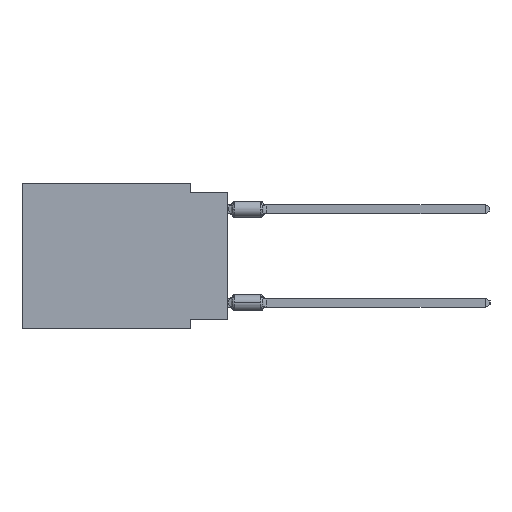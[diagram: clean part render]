
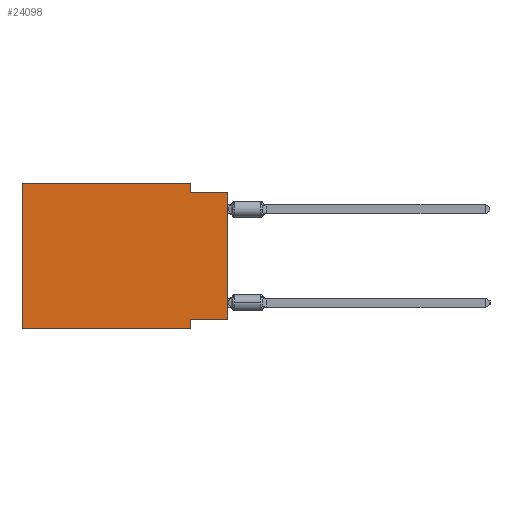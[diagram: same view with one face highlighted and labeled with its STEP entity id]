
A CAD part, left-side view. The second image highlights one B-rep face of the part: STEP entity #24098.
In plain terms, the highlighted planar face has unit normal (-1, 0, 0).
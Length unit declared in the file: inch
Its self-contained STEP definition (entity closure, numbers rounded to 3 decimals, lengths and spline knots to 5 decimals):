
#753 = DIRECTION ( 'NONE',  ( 0., 0., 1. ) ) ;
#770 = ORIENTED_EDGE ( 'NONE', *, *, #48475, .F. ) ;
#1580 = VERTEX_POINT ( 'NONE', #3614 ) ;
#2032 = DIRECTION ( 'NONE',  ( 0., 1., 0. ) ) ;
#2616 = CARTESIAN_POINT ( 'NONE',  ( 0., 0.1, 0. ) ) ;
#3614 = CARTESIAN_POINT ( 'NONE',  ( 0., 0.55, -0.39 ) ) ;
#4252 = ORIENTED_EDGE ( 'NONE', *, *, #18053, .T. ) ;
#5005 = CARTESIAN_POINT ( 'NONE',  ( 0., 0.55, 0. ) ) ;
#5665 = LINE ( 'NONE', #32160, #41641 ) ;
#5710 = ORIENTED_EDGE ( 'NONE', *, *, #48675, .F. ) ;
#7421 = CARTESIAN_POINT ( 'NONE',  ( 0., 0.1, 0. ) ) ;
#7492 = LINE ( 'NONE', #16198, #19968 ) ;
#7508 = VECTOR ( 'NONE', #34671, 39.37008 ) ;
#7801 = ORIENTED_EDGE ( 'NONE', *, *, #20424, .F. ) ;
#8474 = CARTESIAN_POINT ( 'NONE',  ( 0., 0., 0. ) ) ;
#8736 = EDGE_LOOP ( 'NONE', ( #4252, #10594, #26807, #7801, #46024, #19995, #770, #5710 ) ) ;
#9872 = DIRECTION ( 'NONE',  ( 1., 0., 0. ) ) ;
#10594 = ORIENTED_EDGE ( 'NONE', *, *, #32738, .F. ) ;
#10736 = CARTESIAN_POINT ( 'NONE',  ( 0., 0., -0.025 ) ) ;
#11546 = LINE ( 'NONE', #8474, #40232 ) ;
#13713 = PLANE ( 'NONE',  #44706 ) ;
#15048 = VECTOR ( 'NONE', #2032, 39.37008 ) ;
#16198 = CARTESIAN_POINT ( 'NONE',  ( 0., 0.1, -0.39 ) ) ;
#18053 = EDGE_CURVE ( 'NONE', #22342, #47427, #11546, .T. ) ;
#19968 = VECTOR ( 'NONE', #23126, 39.37008 ) ;
#19995 = ORIENTED_EDGE ( 'NONE', *, *, #44096, .T. ) ;
#20424 = EDGE_CURVE ( 'NONE', #35975, #30693, #30299, .T. ) ;
#21227 = CARTESIAN_POINT ( 'NONE',  ( 0., 0., -0.025 ) ) ;
#22306 = DIRECTION ( 'NONE',  ( 0., -1., 0. ) ) ;
#22342 = VERTEX_POINT ( 'NONE', #44874 ) ;
#23126 = DIRECTION ( 'NONE',  ( 0., 0., -1. ) ) ;
#24098 = ADVANCED_FACE ( 'NONE', ( #28638 ), #13713, .F. ) ;
#24459 = VERTEX_POINT ( 'NONE', #33199 ) ;
#25014 = DIRECTION ( 'NONE',  ( 0., 0., -1. ) ) ;
#25878 = LINE ( 'NONE', #10736, #28758 ) ;
#26807 = ORIENTED_EDGE ( 'NONE', *, *, #47073, .F. ) ;
#28638 = FACE_OUTER_BOUND ( 'NONE', #8736, .T. ) ;
#28758 = VECTOR ( 'NONE', #41593, 39.37008 ) ;
#30299 = LINE ( 'NONE', #46009, #34565 ) ;
#30693 = VERTEX_POINT ( 'NONE', #2616 ) ;
#31431 = CARTESIAN_POINT ( 'NONE',  ( 0., 0.1, -0.025 ) ) ;
#32160 = CARTESIAN_POINT ( 'NONE',  ( 0., 0.55, 0. ) ) ;
#32399 = LINE ( 'NONE', #38014, #15048 ) ;
#32738 = EDGE_CURVE ( 'NONE', #37329, #47427, #25878, .T. ) ;
#32834 = VECTOR ( 'NONE', #36633, 39.37008 ) ;
#33199 = CARTESIAN_POINT ( 'NONE',  ( 0., 0.1, -0.39 ) ) ;
#34565 = VECTOR ( 'NONE', #22306, 39.37008 ) ;
#34671 = DIRECTION ( 'NONE',  ( 0., 0., -1. ) ) ;
#35975 = VERTEX_POINT ( 'NONE', #36599 ) ;
#36599 = CARTESIAN_POINT ( 'NONE',  ( 0., 0.55, 0. ) ) ;
#36633 = DIRECTION ( 'NONE',  ( 0., -1., 0. ) ) ;
#37329 = VERTEX_POINT ( 'NONE', #31431 ) ;
#37376 = LINE ( 'NONE', #40266, #32834 ) ;
#38014 = CARTESIAN_POINT ( 'NONE',  ( 0., 0., -0.365 ) ) ;
#38254 = LINE ( 'NONE', #7421, #7508 ) ;
#39060 = EDGE_CURVE ( 'NONE', #1580, #35975, #5665, .T. ) ;
#40232 = VECTOR ( 'NONE', #753, 39.37008 ) ;
#40266 = CARTESIAN_POINT ( 'NONE',  ( 0., 0.55, -0.39 ) ) ;
#41593 = DIRECTION ( 'NONE',  ( 0., -1., 0. ) ) ;
#41641 = VECTOR ( 'NONE', #47854, 39.37008 ) ;
#44096 = EDGE_CURVE ( 'NONE', #1580, #24459, #37376, .T. ) ;
#44706 = AXIS2_PLACEMENT_3D ( 'NONE', #5005, #9872, #25014 ) ;
#44874 = CARTESIAN_POINT ( 'NONE',  ( 0., 0., -0.365 ) ) ;
#46009 = CARTESIAN_POINT ( 'NONE',  ( 0., 0.55, 0. ) ) ;
#46024 = ORIENTED_EDGE ( 'NONE', *, *, #39060, .F. ) ;
#47073 = EDGE_CURVE ( 'NONE', #30693, #37329, #38254, .T. ) ;
#47427 = VERTEX_POINT ( 'NONE', #21227 ) ;
#47752 = VERTEX_POINT ( 'NONE', #48968 ) ;
#47854 = DIRECTION ( 'NONE',  ( 0., 0., 1. ) ) ;
#48475 = EDGE_CURVE ( 'NONE', #47752, #24459, #7492, .T. ) ;
#48675 = EDGE_CURVE ( 'NONE', #22342, #47752, #32399, .T. ) ;
#48968 = CARTESIAN_POINT ( 'NONE',  ( 0., 0.1, -0.365 ) ) ;
